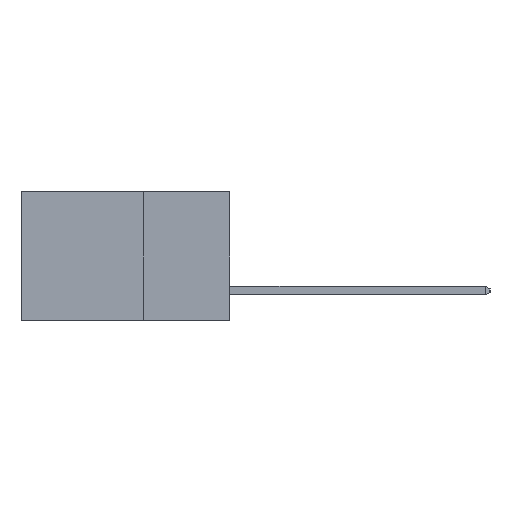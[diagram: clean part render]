
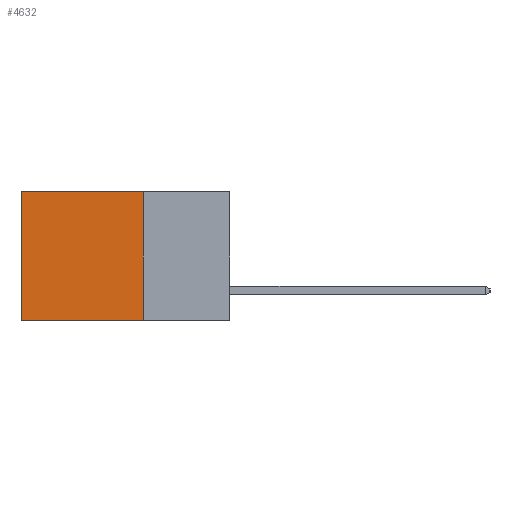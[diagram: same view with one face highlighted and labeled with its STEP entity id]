
A CAD part, left-side view. The second image highlights one B-rep face of the part: STEP entity #4632.
In plain terms, the highlighted planar face has unit normal (-1, 0, 0).
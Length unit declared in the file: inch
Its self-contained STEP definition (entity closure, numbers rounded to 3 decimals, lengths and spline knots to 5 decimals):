
#716 = VECTOR ( 'NONE', #9579, 39.37008 ) ;
#1007 = CARTESIAN_POINT ( 'NONE',  ( 0.2615, 0.25, -0.37 ) ) ;
#1343 = FACE_OUTER_BOUND ( 'NONE', #3181, .T. ) ;
#1584 = ORIENTED_EDGE ( 'NONE', *, *, #9365, .F. ) ;
#1629 = VERTEX_POINT ( 'NONE', #9999 ) ;
#2206 = ORIENTED_EDGE ( 'NONE', *, *, #5577, .T. ) ;
#3181 = EDGE_LOOP ( 'NONE', ( #6537, #4941, #1584, #2206 ) ) ;
#3495 = CARTESIAN_POINT ( 'NONE',  ( 0.2615, 0.25, -0.37 ) ) ;
#4124 = VECTOR ( 'NONE', #8785, 39.37008 ) ;
#4203 = DIRECTION ( 'NONE',  ( 1., 0., 0. ) ) ;
#4632 = ADVANCED_FACE ( 'NONE', ( #1343 ), #9178, .F. ) ;
#4941 = ORIENTED_EDGE ( 'NONE', *, *, #11290, .F. ) ;
#5577 = EDGE_CURVE ( 'NONE', #1629, #10126, #12148, .T. ) ;
#5733 = LINE ( 'NONE', #3495, #10703 ) ;
#5817 = CARTESIAN_POINT ( 'NONE',  ( 0.2615, 0.25, 0. ) ) ;
#5884 = EDGE_CURVE ( 'NONE', #10126, #8769, #8088, .T. ) ;
#6329 = LINE ( 'NONE', #8600, #716 ) ;
#6537 = ORIENTED_EDGE ( 'NONE', *, *, #5884, .T. ) ;
#7853 = DIRECTION ( 'NONE',  ( 0., 0., -1. ) ) ;
#8088 = LINE ( 'NONE', #12811, #10715 ) ;
#8600 = CARTESIAN_POINT ( 'NONE',  ( 0.2615, 0.25, -0.37 ) ) ;
#8769 = VERTEX_POINT ( 'NONE', #11502 ) ;
#8785 = DIRECTION ( 'NONE',  ( 0., 1., 0. ) ) ;
#9178 = PLANE ( 'NONE',  #10378 ) ;
#9365 = EDGE_CURVE ( 'NONE', #1629, #12851, #6329, .T. ) ;
#9579 = DIRECTION ( 'NONE',  ( 0., 0., -1. ) ) ;
#9637 = CARTESIAN_POINT ( 'NONE',  ( 0.2615, 0.25, -0.37 ) ) ;
#9999 = CARTESIAN_POINT ( 'NONE',  ( 0.2615, 0.25, 0. ) ) ;
#10126 = VERTEX_POINT ( 'NONE', #11781 ) ;
#10378 = AXIS2_PLACEMENT_3D ( 'NONE', #1007, #4203, #11241 ) ;
#10703 = VECTOR ( 'NONE', #11568, 39.37008 ) ;
#10715 = VECTOR ( 'NONE', #7853, 39.37008 ) ;
#11241 = DIRECTION ( 'NONE',  ( 0., 0., -1. ) ) ;
#11290 = EDGE_CURVE ( 'NONE', #12851, #8769, #5733, .T. ) ;
#11502 = CARTESIAN_POINT ( 'NONE',  ( 0.2615, 0.6, -0.37 ) ) ;
#11568 = DIRECTION ( 'NONE',  ( 0., 1., 0. ) ) ;
#11781 = CARTESIAN_POINT ( 'NONE',  ( 0.2615, 0.6, 0. ) ) ;
#12148 = LINE ( 'NONE', #5817, #4124 ) ;
#12811 = CARTESIAN_POINT ( 'NONE',  ( 0.2615, 0.6, -0.37 ) ) ;
#12851 = VERTEX_POINT ( 'NONE', #9637 ) ;
